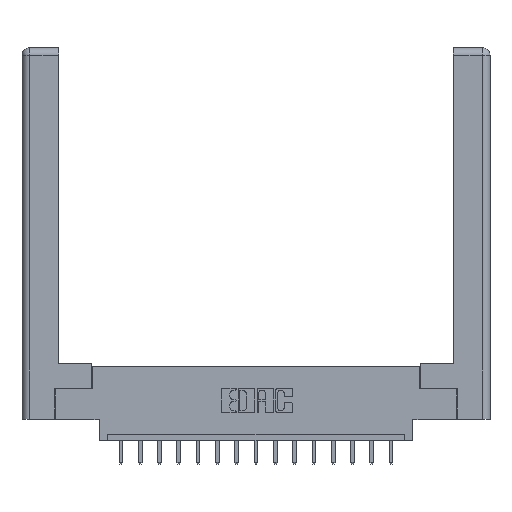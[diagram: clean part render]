
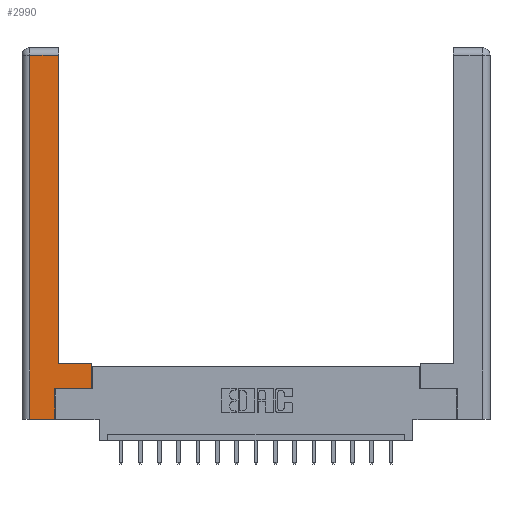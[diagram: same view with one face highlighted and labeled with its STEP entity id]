
A CAD part, top view. The second image highlights one B-rep face of the part: STEP entity #2990.
In plain terms, the highlighted planar face has unit normal (0, 0, 1).
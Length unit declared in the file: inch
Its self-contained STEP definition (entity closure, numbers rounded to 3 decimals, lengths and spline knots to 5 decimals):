
#87 = PLANE ( 'NONE',  #1955 ) ;
#312 = VECTOR ( 'NONE', #15071, 39.37008 ) ;
#396 = VERTEX_POINT ( 'NONE', #1628 ) ;
#784 = CARTESIAN_POINT ( 'NONE',  ( 0., 0., 0. ) ) ;
#1628 = CARTESIAN_POINT ( 'NONE',  ( 0.565, 0.245, 0. ) ) ;
#1673 = ORIENTED_EDGE ( 'NONE', *, *, #7925, .T. ) ;
#1922 = DIRECTION ( 'NONE',  ( 0., 1., 0. ) ) ;
#1955 = AXIS2_PLACEMENT_3D ( 'NONE', #784, #3385, #15716 ) ;
#2018 = DIRECTION ( 'NONE',  ( 1., 0., 0. ) ) ;
#2247 = VERTEX_POINT ( 'NONE', #12644 ) ;
#2714 = CARTESIAN_POINT ( 'NONE',  ( 0.265, 0., 0. ) ) ;
#2847 = ORIENTED_EDGE ( 'NONE', *, *, #7573, .T. ) ;
#2864 = FACE_OUTER_BOUND ( 'NONE', #14929, .T. ) ;
#2972 = DIRECTION ( 'NONE',  ( 0., 1., 0. ) ) ;
#2990 = ADVANCED_FACE ( 'NONE', ( #2864 ), #87, .F. ) ;
#3090 = ORIENTED_EDGE ( 'NONE', *, *, #14909, .T. ) ;
#3301 = VECTOR ( 'NONE', #1922, 39.37008 ) ;
#3385 = DIRECTION ( 'NONE',  ( 0., 0., -1. ) ) ;
#3438 = VECTOR ( 'NONE', #10865, 39.37008 ) ;
#3503 = LINE ( 'NONE', #15764, #7347 ) ;
#3652 = LINE ( 'NONE', #6258, #9427 ) ;
#4285 = LINE ( 'NONE', #7425, #12360 ) ;
#5046 = VERTEX_POINT ( 'NONE', #7629 ) ;
#5533 = CARTESIAN_POINT ( 'NONE',  ( 0.0615, 0., 0. ) ) ;
#5858 = ORIENTED_EDGE ( 'NONE', *, *, #16783, .T. ) ;
#6253 = DIRECTION ( 'NONE',  ( -1., 0., 0. ) ) ;
#6258 = CARTESIAN_POINT ( 'NONE',  ( 0.265, 0., 0. ) ) ;
#6749 = CARTESIAN_POINT ( 'NONE',  ( 0.565, 0.245, 0. ) ) ;
#6890 = LINE ( 'NONE', #11140, #12099 ) ;
#7129 = LINE ( 'NONE', #6749, #312 ) ;
#7347 = VECTOR ( 'NONE', #6253, 39.37008 ) ;
#7404 = CARTESIAN_POINT ( 'NONE',  ( 0.565, 0.45, 0. ) ) ;
#7425 = CARTESIAN_POINT ( 'NONE',  ( 0.265, 0.245, 0. ) ) ;
#7573 = EDGE_CURVE ( 'NONE', #9608, #2247, #3503, .T. ) ;
#7606 = ORIENTED_EDGE ( 'NONE', *, *, #17179, .T. ) ;
#7629 = CARTESIAN_POINT ( 'NONE',  ( 0.0615, 2.94, 0. ) ) ;
#7807 = LINE ( 'NONE', #7404, #3301 ) ;
#7925 = EDGE_CURVE ( 'NONE', #11036, #396, #7129, .T. ) ;
#8412 = ORIENTED_EDGE ( 'NONE', *, *, #16625, .T. ) ;
#8979 = DIRECTION ( 'NONE',  ( 0., 1., 0. ) ) ;
#9427 = VECTOR ( 'NONE', #2018, 39.37008 ) ;
#9511 = CARTESIAN_POINT ( 'NONE',  ( 0.565, 0.45, 0. ) ) ;
#9582 = LINE ( 'NONE', #5533, #14195 ) ;
#9608 = VERTEX_POINT ( 'NONE', #9511 ) ;
#9624 = LINE ( 'NONE', #14637, #3438 ) ;
#9697 = DIRECTION ( 'NONE',  ( 0., -1., 0. ) ) ;
#10865 = DIRECTION ( 'NONE',  ( -1., 0., 0. ) ) ;
#10890 = ORIENTED_EDGE ( 'NONE', *, *, #10923, .T. ) ;
#10923 = EDGE_CURVE ( 'NONE', #5046, #15861, #9582, .T. ) ;
#11036 = VERTEX_POINT ( 'NONE', #13912 ) ;
#11140 = CARTESIAN_POINT ( 'NONE',  ( 0.295, 3., 0. ) ) ;
#12099 = VECTOR ( 'NONE', #2972, 39.37008 ) ;
#12360 = VECTOR ( 'NONE', #8979, 39.37008 ) ;
#12400 = CARTESIAN_POINT ( 'NONE',  ( 0.0615, 0., 0. ) ) ;
#12644 = CARTESIAN_POINT ( 'NONE',  ( 0.295, 0.45, 0. ) ) ;
#13526 = EDGE_CURVE ( 'NONE', #2247, #17146, #6890, .T. ) ;
#13912 = CARTESIAN_POINT ( 'NONE',  ( 0.265, 0.245, 0. ) ) ;
#14145 = CARTESIAN_POINT ( 'NONE',  ( 0.295, 2.94, 0. ) ) ;
#14195 = VECTOR ( 'NONE', #9697, 39.37008 ) ;
#14637 = CARTESIAN_POINT ( 'NONE',  ( 0.0615, 2.94, 0. ) ) ;
#14909 = EDGE_CURVE ( 'NONE', #396, #9608, #7807, .T. ) ;
#14929 = EDGE_LOOP ( 'NONE', ( #16181, #5858, #10890, #8412, #7606, #1673, #3090, #2847 ) ) ;
#15071 = DIRECTION ( 'NONE',  ( 1., 0., 0. ) ) ;
#15716 = DIRECTION ( 'NONE',  ( -1., 0., 0. ) ) ;
#15764 = CARTESIAN_POINT ( 'NONE',  ( 0.295, 0.45, 0. ) ) ;
#15861 = VERTEX_POINT ( 'NONE', #12400 ) ;
#16181 = ORIENTED_EDGE ( 'NONE', *, *, #13526, .T. ) ;
#16625 = EDGE_CURVE ( 'NONE', #15861, #16890, #3652, .T. ) ;
#16783 = EDGE_CURVE ( 'NONE', #17146, #5046, #9624, .T. ) ;
#16890 = VERTEX_POINT ( 'NONE', #2714 ) ;
#17146 = VERTEX_POINT ( 'NONE', #14145 ) ;
#17179 = EDGE_CURVE ( 'NONE', #16890, #11036, #4285, .T. ) ;
